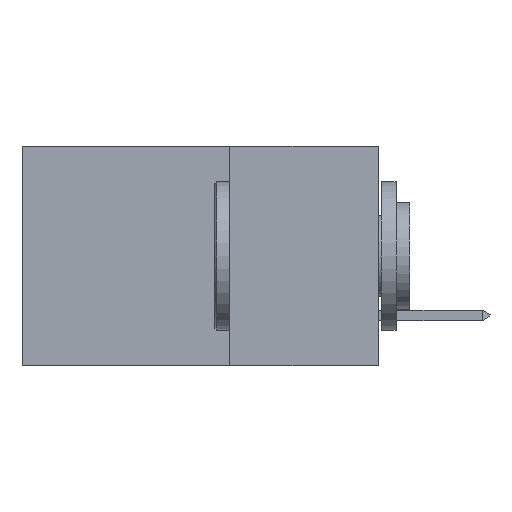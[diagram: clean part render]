
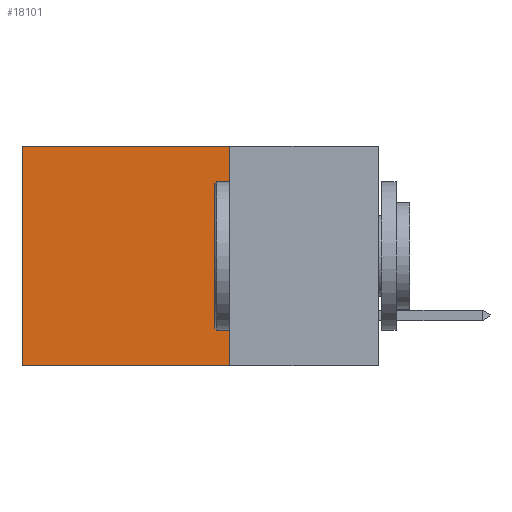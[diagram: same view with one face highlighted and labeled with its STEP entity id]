
A CAD part, left-side view. The second image highlights one B-rep face of the part: STEP entity #18101.
In plain terms, the highlighted planar face has unit normal (-1, 0, 0).
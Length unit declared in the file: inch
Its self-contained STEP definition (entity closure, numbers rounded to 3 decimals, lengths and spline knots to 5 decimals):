
#1182 = CARTESIAN_POINT ( 'NONE',  ( 0.298, 0.25, -0.37 ) ) ;
#2547 = EDGE_CURVE ( 'NONE', #22000, #22283, #17453, .T. ) ;
#3620 = EDGE_CURVE ( 'NONE', #11920, #22283, #6771, .T. ) ;
#3825 = LINE ( 'NONE', #19445, #13736 ) ;
#4769 = ORIENTED_EDGE ( 'NONE', *, *, #3620, .F. ) ;
#5242 = DIRECTION ( 'NONE',  ( 1., 0., 0. ) ) ;
#5311 = EDGE_CURVE ( 'NONE', #24526, #11920, #3825, .T. ) ;
#5436 = CARTESIAN_POINT ( 'NONE',  ( 0.298, 0.6, 0. ) ) ;
#5589 = DIRECTION ( 'NONE',  ( 0., 0., -1. ) ) ;
#6684 = CARTESIAN_POINT ( 'NONE',  ( 0.298, 0.25, -0.37 ) ) ;
#6771 = LINE ( 'NONE', #6684, #10313 ) ;
#7437 = PLANE ( 'NONE',  #27709 ) ;
#8956 = DIRECTION ( 'NONE',  ( 0., 1., 0. ) ) ;
#10313 = VECTOR ( 'NONE', #8956, 39.37008 ) ;
#11920 = VERTEX_POINT ( 'NONE', #1182 ) ;
#12258 = CARTESIAN_POINT ( 'NONE',  ( 0.298, 0.6, 0. ) ) ;
#12639 = DIRECTION ( 'NONE',  ( 0., 0., -1. ) ) ;
#13707 = ORIENTED_EDGE ( 'NONE', *, *, #5311, .F. ) ;
#13736 = VECTOR ( 'NONE', #5589, 39.37008 ) ;
#16575 = ORIENTED_EDGE ( 'NONE', *, *, #23781, .T. ) ;
#16718 = VECTOR ( 'NONE', #12639, 39.37008 ) ;
#16780 = CARTESIAN_POINT ( 'NONE',  ( 0.298, 0.6, -0.37 ) ) ;
#16934 = CARTESIAN_POINT ( 'NONE',  ( 0.298, 0.25, 0. ) ) ;
#17453 = LINE ( 'NONE', #12258, #16718 ) ;
#18101 = ADVANCED_FACE ( 'NONE', ( #18814 ), #7437, .F. ) ;
#18361 = ORIENTED_EDGE ( 'NONE', *, *, #2547, .T. ) ;
#18814 = FACE_OUTER_BOUND ( 'NONE', #28440, .T. ) ;
#19445 = CARTESIAN_POINT ( 'NONE',  ( 0.298, 0.25, 0. ) ) ;
#20940 = DIRECTION ( 'NONE',  ( 0., 1., 0. ) ) ;
#21996 = VECTOR ( 'NONE', #20940, 39.37008 ) ;
#22000 = VERTEX_POINT ( 'NONE', #5436 ) ;
#22283 = VERTEX_POINT ( 'NONE', #16780 ) ;
#23354 = CARTESIAN_POINT ( 'NONE',  ( 0.298, 0.25, 0. ) ) ;
#23781 = EDGE_CURVE ( 'NONE', #24526, #22000, #24846, .T. ) ;
#24365 = CARTESIAN_POINT ( 'NONE',  ( 0.298, 0.25, 0. ) ) ;
#24526 = VERTEX_POINT ( 'NONE', #24365 ) ;
#24846 = LINE ( 'NONE', #23354, #21996 ) ;
#27709 = AXIS2_PLACEMENT_3D ( 'NONE', #16934, #5242, #28231 ) ;
#28231 = DIRECTION ( 'NONE',  ( 0., 0., -1. ) ) ;
#28440 = EDGE_LOOP ( 'NONE', ( #18361, #4769, #13707, #16575 ) ) ;
